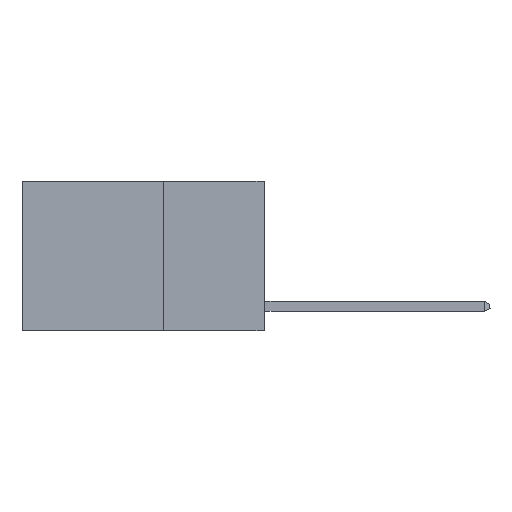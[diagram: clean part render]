
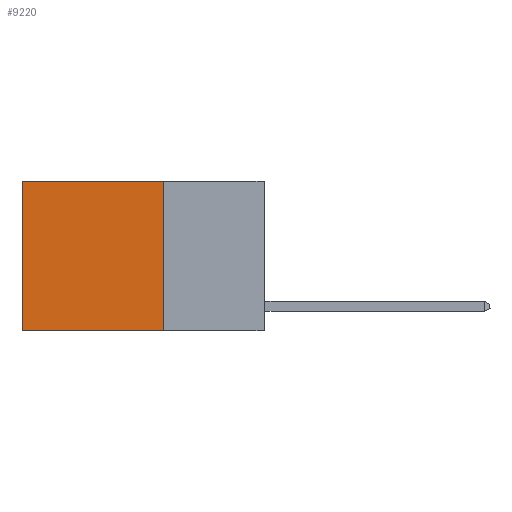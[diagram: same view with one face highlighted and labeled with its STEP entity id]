
A CAD part, left-side view. The second image highlights one B-rep face of the part: STEP entity #9220.
In plain terms, the highlighted planar face has unit normal (-1, 0, 0).
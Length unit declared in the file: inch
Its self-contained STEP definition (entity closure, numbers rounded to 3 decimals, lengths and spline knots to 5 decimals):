
#233 = CARTESIAN_POINT ( 'NONE',  ( 0.2625, 0.25, -0.37 ) ) ;
#528 = LINE ( 'NONE', #4419, #1727 ) ;
#932 = DIRECTION ( 'NONE',  ( 0., 0., -1. ) ) ;
#1105 = VECTOR ( 'NONE', #22194, 39.37008 ) ;
#1197 = EDGE_CURVE ( 'NONE', #12429, #13273, #528, .T. ) ;
#1344 = CARTESIAN_POINT ( 'NONE',  ( 0.2625, 0.25, -0.37 ) ) ;
#1592 = AXIS2_PLACEMENT_3D ( 'NONE', #12929, #11256, #932 ) ;
#1727 = VECTOR ( 'NONE', #7887, 39.37008 ) ;
#2094 = CARTESIAN_POINT ( 'NONE',  ( 0.2625, 0.25, 0. ) ) ;
#3114 = ORIENTED_EDGE ( 'NONE', *, *, #21225, .F. ) ;
#3169 = CARTESIAN_POINT ( 'NONE',  ( 0.2625, 0.6, 0. ) ) ;
#3391 = ORIENTED_EDGE ( 'NONE', *, *, #6042, .T. ) ;
#3870 = LINE ( 'NONE', #1344, #8501 ) ;
#4419 = CARTESIAN_POINT ( 'NONE',  ( 0.2625, 0.6, 0. ) ) ;
#6042 = EDGE_CURVE ( 'NONE', #13147, #12429, #6661, .T. ) ;
#6661 = LINE ( 'NONE', #2094, #19267 ) ;
#7470 = CARTESIAN_POINT ( 'NONE',  ( 0.2625, 0.6, -0.37 ) ) ;
#7887 = DIRECTION ( 'NONE',  ( 0., 0., -1. ) ) ;
#8501 = VECTOR ( 'NONE', #11675, 39.37008 ) ;
#9057 = DIRECTION ( 'NONE',  ( 0., 1., 0. ) ) ;
#9220 = ADVANCED_FACE ( 'NONE', ( #20567 ), #21470, .F. ) ;
#10042 = EDGE_CURVE ( 'NONE', #21341, #13273, #3870, .T. ) ;
#10292 = CARTESIAN_POINT ( 'NONE',  ( 0.2625, 0.25, 0. ) ) ;
#10301 = LINE ( 'NONE', #10292, #1105 ) ;
#11256 = DIRECTION ( 'NONE',  ( 1., 0., 0. ) ) ;
#11675 = DIRECTION ( 'NONE',  ( 0., 1., 0. ) ) ;
#12429 = VERTEX_POINT ( 'NONE', #3169 ) ;
#12929 = CARTESIAN_POINT ( 'NONE',  ( 0.2625, 0.25, 0. ) ) ;
#13147 = VERTEX_POINT ( 'NONE', #17410 ) ;
#13273 = VERTEX_POINT ( 'NONE', #7470 ) ;
#16436 = ORIENTED_EDGE ( 'NONE', *, *, #1197, .T. ) ;
#17410 = CARTESIAN_POINT ( 'NONE',  ( 0.2625, 0.25, 0. ) ) ;
#17798 = ORIENTED_EDGE ( 'NONE', *, *, #10042, .F. ) ;
#19267 = VECTOR ( 'NONE', #9057, 39.37008 ) ;
#20567 = FACE_OUTER_BOUND ( 'NONE', #20761, .T. ) ;
#20761 = EDGE_LOOP ( 'NONE', ( #16436, #17798, #3114, #3391 ) ) ;
#21225 = EDGE_CURVE ( 'NONE', #13147, #21341, #10301, .T. ) ;
#21341 = VERTEX_POINT ( 'NONE', #233 ) ;
#21470 = PLANE ( 'NONE',  #1592 ) ;
#22194 = DIRECTION ( 'NONE',  ( 0., 0., -1. ) ) ;
